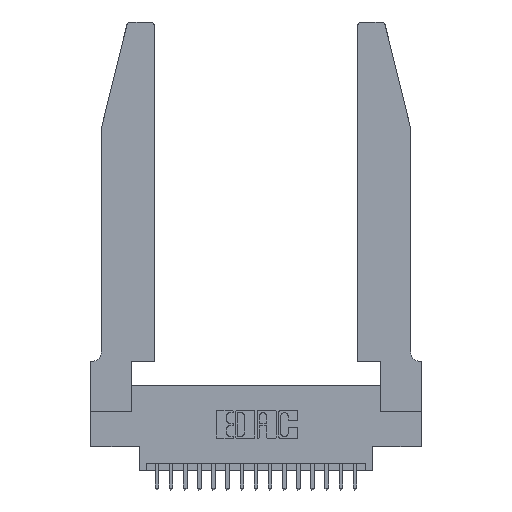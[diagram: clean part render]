
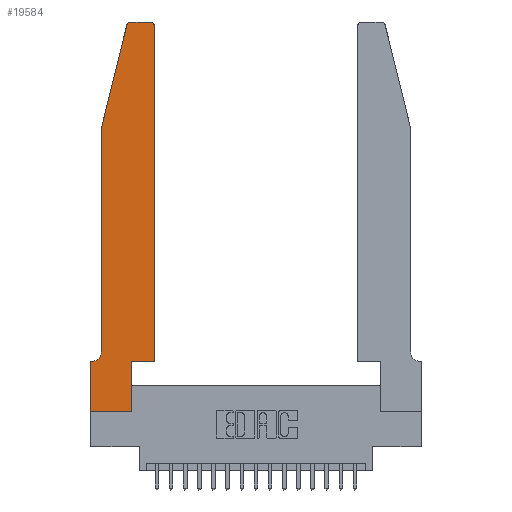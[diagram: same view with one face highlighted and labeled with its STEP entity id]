
A CAD part, top view. The second image highlights one B-rep face of the part: STEP entity #19584.
In plain terms, the highlighted planar face has unit normal (0, 0, 1).
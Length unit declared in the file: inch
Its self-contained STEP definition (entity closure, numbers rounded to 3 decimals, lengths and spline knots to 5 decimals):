
#16 = CARTESIAN_POINT ( 'NONE',  ( 0., 0.35, 0.37 ) ) ;
#48 = LINE ( 'NONE', #14948, #7977 ) ;
#301 = EDGE_CURVE ( 'NONE', #2702, #6601, #11011, .T. ) ;
#397 = VERTEX_POINT ( 'NONE', #18502 ) ;
#740 = VECTOR ( 'NONE', #7535, 39.37008 ) ;
#1259 = CARTESIAN_POINT ( 'NONE',  ( 0.0755, 2., 0.37 ) ) ;
#1308 = ORIENTED_EDGE ( 'NONE', *, *, #3356, .T. ) ;
#1323 = CARTESIAN_POINT ( 'NONE',  ( 0., 0.35, 0.37 ) ) ;
#1410 = AXIS2_PLACEMENT_3D ( 'NONE', #6809, #12551, #20328 ) ;
#1523 = CARTESIAN_POINT ( 'NONE',  ( 0., 0., 0.37 ) ) ;
#1573 = ORIENTED_EDGE ( 'NONE', *, *, #16886, .T. ) ;
#2082 = ORIENTED_EDGE ( 'NONE', *, *, #8115, .T. ) ;
#2285 = CARTESIAN_POINT ( 'NONE',  ( 0.2865, 0., 0.37 ) ) ;
#2364 = DIRECTION ( 'NONE',  ( -1., 0., 0. ) ) ;
#2426 = DIRECTION ( 'NONE',  ( 0., 1., 0. ) ) ;
#2694 = EDGE_CURVE ( 'NONE', #6601, #10772, #16623, .T. ) ;
#2702 = VERTEX_POINT ( 'NONE', #6580 ) ;
#2723 = VERTEX_POINT ( 'NONE', #6828 ) ;
#2915 = DIRECTION ( 'NONE',  ( 1., 0., 0. ) ) ;
#3356 = EDGE_CURVE ( 'NONE', #17476, #397, #5293, .T. ) ;
#3869 = CARTESIAN_POINT ( 'NONE',  ( 0.0755, 2., 0.37 ) ) ;
#3934 = EDGE_CURVE ( 'NONE', #10772, #2723, #48, .T. ) ;
#4001 = CARTESIAN_POINT ( 'NONE',  ( 0., 0., 0.37 ) ) ;
#4556 = ORIENTED_EDGE ( 'NONE', *, *, #17778, .T. ) ;
#4969 = LINE ( 'NONE', #1259, #740 ) ;
#5046 = ORIENTED_EDGE ( 'NONE', *, *, #15605, .T. ) ;
#5195 = VECTOR ( 'NONE', #10524, 39.37008 ) ;
#5293 = CIRCLE ( 'NONE', #19899, 0.07 ) ;
#5472 = EDGE_CURVE ( 'NONE', #11490, #15173, #4969, .T. ) ;
#5905 = CARTESIAN_POINT ( 'NONE',  ( 0.0055, 0.42, 0.37 ) ) ;
#6249 = DIRECTION ( 'NONE',  ( -1., 0., 0. ) ) ;
#6580 = CARTESIAN_POINT ( 'NONE',  ( 0.4505, 0.35, 0.37 ) ) ;
#6601 = VERTEX_POINT ( 'NONE', #7843 ) ;
#6647 = CARTESIAN_POINT ( 'NONE',  ( 0.0755, 2., 0.37 ) ) ;
#6809 = CARTESIAN_POINT ( 'NONE',  ( 0.4205, 2.72, 0.37 ) ) ;
#6828 = CARTESIAN_POINT ( 'NONE',  ( 0.284, 2.75, 0.37 ) ) ;
#6832 = VECTOR ( 'NONE', #16598, 39.37008 ) ;
#7143 = DIRECTION ( 'NONE',  ( -1., 0., 0. ) ) ;
#7164 = CIRCLE ( 'NONE', #9756, 0.03 ) ;
#7181 = DIRECTION ( 'NONE',  ( 0., 0., -1. ) ) ;
#7525 = DIRECTION ( 'NONE',  ( 0., 0., 1. ) ) ;
#7535 = DIRECTION ( 'NONE',  ( -0.239, -0.971, 0. ) ) ;
#7544 = VECTOR ( 'NONE', #13993, 39.37008 ) ;
#7843 = CARTESIAN_POINT ( 'NONE',  ( 0.4505, 2.72, 0.37 ) ) ;
#7977 = VECTOR ( 'NONE', #2364, 39.37008 ) ;
#8061 = VERTEX_POINT ( 'NONE', #2285 ) ;
#8115 = EDGE_CURVE ( 'NONE', #16375, #13686, #15620, .T. ) ;
#8510 = LINE ( 'NONE', #3869, #12209 ) ;
#9756 = AXIS2_PLACEMENT_3D ( 'NONE', #16935, #7525, #18485 ) ;
#9924 = EDGE_LOOP ( 'NONE', ( #13617, #18253, #18735, #17055, #1308, #1573, #2082, #14625, #4556, #5046, #15375, #12175 ) ) ;
#10029 = EDGE_CURVE ( 'NONE', #2723, #11490, #7164, .T. ) ;
#10401 = LINE ( 'NONE', #19511, #18721 ) ;
#10524 = DIRECTION ( 'NONE',  ( 1., 0., 0. ) ) ;
#10610 = EDGE_CURVE ( 'NONE', #13686, #8061, #14051, .T. ) ;
#10772 = VERTEX_POINT ( 'NONE', #15547 ) ;
#10817 = CARTESIAN_POINT ( 'NONE',  ( 0.4505, 0.35, 0.37 ) ) ;
#11011 = LINE ( 'NONE', #14193, #6832 ) ;
#11490 = VERTEX_POINT ( 'NONE', #18834 ) ;
#11705 = DIRECTION ( 'NONE',  ( 0., -1., 0. ) ) ;
#12175 = ORIENTED_EDGE ( 'NONE', *, *, #2694, .T. ) ;
#12209 = VECTOR ( 'NONE', #11705, 39.37008 ) ;
#12347 = DIRECTION ( 'NONE',  ( 0., 0., 1. ) ) ;
#12492 = CARTESIAN_POINT ( 'NONE',  ( 0.0755, 0.35, 0.37 ) ) ;
#12551 = DIRECTION ( 'NONE',  ( 0., 0., 1. ) ) ;
#13142 = VECTOR ( 'NONE', #6249, 39.37008 ) ;
#13617 = ORIENTED_EDGE ( 'NONE', *, *, #3934, .T. ) ;
#13637 = LINE ( 'NONE', #12492, #13142 ) ;
#13686 = VERTEX_POINT ( 'NONE', #1523 ) ;
#13993 = DIRECTION ( 'NONE',  ( 1., 0., 0. ) ) ;
#14018 = EDGE_CURVE ( 'NONE', #15173, #17476, #8510, .T. ) ;
#14051 = LINE ( 'NONE', #18325, #5195 ) ;
#14193 = CARTESIAN_POINT ( 'NONE',  ( 0.4505, 0.35, 0.37 ) ) ;
#14607 = VERTEX_POINT ( 'NONE', #16470 ) ;
#14625 = ORIENTED_EDGE ( 'NONE', *, *, #10610, .T. ) ;
#14948 = CARTESIAN_POINT ( 'NONE',  ( 0.2605, 2.75, 0.37 ) ) ;
#15173 = VERTEX_POINT ( 'NONE', #6647 ) ;
#15375 = ORIENTED_EDGE ( 'NONE', *, *, #301, .T. ) ;
#15547 = CARTESIAN_POINT ( 'NONE',  ( 0.4205, 2.75, 0.37 ) ) ;
#15605 = EDGE_CURVE ( 'NONE', #14607, #2702, #19987, .T. ) ;
#15620 = LINE ( 'NONE', #4001, #18763 ) ;
#15707 = CARTESIAN_POINT ( 'NONE',  ( 0.0755, 0.42, 0.37 ) ) ;
#16259 = FACE_OUTER_BOUND ( 'NONE', #9924, .T. ) ;
#16375 = VERTEX_POINT ( 'NONE', #16 ) ;
#16470 = CARTESIAN_POINT ( 'NONE',  ( 0.2865, 0.35, 0.37 ) ) ;
#16560 = DIRECTION ( 'NONE',  ( 0., -1., 0. ) ) ;
#16598 = DIRECTION ( 'NONE',  ( 0., 1., 0. ) ) ;
#16623 = CIRCLE ( 'NONE', #1410, 0.03 ) ;
#16886 = EDGE_CURVE ( 'NONE', #397, #16375, #13637, .T. ) ;
#16935 = CARTESIAN_POINT ( 'NONE',  ( 0.284, 2.72, 0.37 ) ) ;
#17055 = ORIENTED_EDGE ( 'NONE', *, *, #14018, .T. ) ;
#17348 = AXIS2_PLACEMENT_3D ( 'NONE', #1323, #12347, #2915 ) ;
#17476 = VERTEX_POINT ( 'NONE', #15707 ) ;
#17778 = EDGE_CURVE ( 'NONE', #8061, #14607, #10401, .T. ) ;
#18253 = ORIENTED_EDGE ( 'NONE', *, *, #10029, .T. ) ;
#18325 = CARTESIAN_POINT ( 'NONE',  ( 0., 0., 0.37 ) ) ;
#18485 = DIRECTION ( 'NONE',  ( 1., 0., 0. ) ) ;
#18502 = CARTESIAN_POINT ( 'NONE',  ( 0.0055, 0.35, 0.37 ) ) ;
#18559 = PLANE ( 'NONE',  #17348 ) ;
#18721 = VECTOR ( 'NONE', #2426, 39.37008 ) ;
#18735 = ORIENTED_EDGE ( 'NONE', *, *, #5472, .T. ) ;
#18763 = VECTOR ( 'NONE', #16560, 39.37008 ) ;
#18834 = CARTESIAN_POINT ( 'NONE',  ( 0.25487, 2.72718, 0.37 ) ) ;
#19511 = CARTESIAN_POINT ( 'NONE',  ( 0.2865, 0.35, 0.37 ) ) ;
#19584 = ADVANCED_FACE ( 'NONE', ( #16259 ), #18559, .T. ) ;
#19899 = AXIS2_PLACEMENT_3D ( 'NONE', #5905, #7181, #7143 ) ;
#19987 = LINE ( 'NONE', #10817, #7544 ) ;
#20328 = DIRECTION ( 'NONE',  ( 1., 0., 0. ) ) ;
